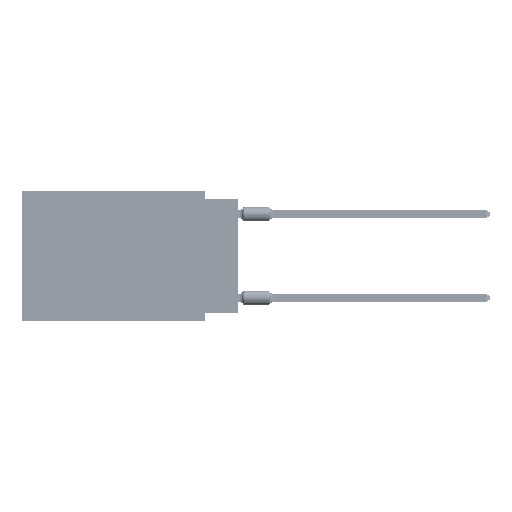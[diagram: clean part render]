
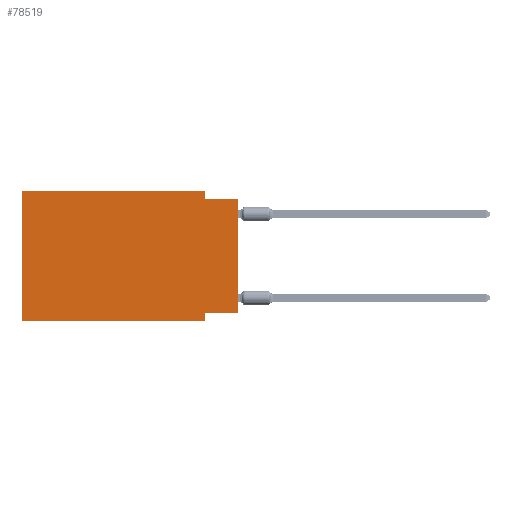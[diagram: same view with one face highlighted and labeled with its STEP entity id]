
A CAD part, left-side view. The second image highlights one B-rep face of the part: STEP entity #78519.
In plain terms, the highlighted planar face has unit normal (-1, 0, 0).
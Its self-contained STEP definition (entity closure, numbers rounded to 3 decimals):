
#569 = EDGE_CURVE ( 'NONE', #36816, #36761, #24789, .T. ) ;
#1434 = LINE ( 'NONE', #35737, #56379 ) ;
#3275 = DIRECTION ( 'NONE',  ( 0., 0., 1. ) ) ;
#5241 = DIRECTION ( 'NONE',  ( 0., 0., -1. ) ) ;
#5574 = ORIENTED_EDGE ( 'NONE', *, *, #16453, .F. ) ;
#5767 = CARTESIAN_POINT ( 'NONE',  ( 0., 0., -9.271 ) ) ;
#7867 = VERTEX_POINT ( 'NONE', #12869 ) ;
#8381 = CARTESIAN_POINT ( 'NONE',  ( 0., 0., -0.635 ) ) ;
#12153 = EDGE_LOOP ( 'NONE', ( #39560, #37066, #29864, #5574, #66683, #27872, #53788, #54369 ) ) ;
#12277 = FACE_OUTER_BOUND ( 'NONE', #12153, .T. ) ;
#12869 = CARTESIAN_POINT ( 'NONE',  ( 0., 16.383, 0. ) ) ;
#13129 = DIRECTION ( 'NONE',  ( 1., 0., 0. ) ) ;
#14637 = DIRECTION ( 'NONE',  ( 0., -1., 0. ) ) ;
#14796 = DIRECTION ( 'NONE',  ( 0., 0., -1. ) ) ;
#16453 = EDGE_CURVE ( 'NONE', #7867, #36816, #38893, .T. ) ;
#18211 = CARTESIAN_POINT ( 'NONE',  ( 0., 2.54, -0.635 ) ) ;
#20026 = EDGE_CURVE ( 'NONE', #57090, #71826, #1434, .T. ) ;
#21146 = CARTESIAN_POINT ( 'NONE',  ( 0., 2.54, -9.271 ) ) ;
#22377 = CARTESIAN_POINT ( 'NONE',  ( 0., 16.383, 0. ) ) ;
#23449 = LINE ( 'NONE', #74256, #75177 ) ;
#24789 = LINE ( 'NONE', #51705, #27773 ) ;
#25863 = CARTESIAN_POINT ( 'NONE',  ( 0., 0., -0.635 ) ) ;
#26068 = CARTESIAN_POINT ( 'NONE',  ( 0., 16.383, -9.906 ) ) ;
#27773 = VECTOR ( 'NONE', #5241, 1000. ) ;
#27872 = ORIENTED_EDGE ( 'NONE', *, *, #71903, .T. ) ;
#28178 = AXIS2_PLACEMENT_3D ( 'NONE', #47009, #13129, #39643 ) ;
#29864 = ORIENTED_EDGE ( 'NONE', *, *, #569, .F. ) ;
#30706 = VERTEX_POINT ( 'NONE', #61162 ) ;
#34869 = DIRECTION ( 'NONE',  ( 0., -1., 0. ) ) ;
#35737 = CARTESIAN_POINT ( 'NONE',  ( 0., 0., -9.271 ) ) ;
#36761 = VERTEX_POINT ( 'NONE', #18211 ) ;
#36816 = VERTEX_POINT ( 'NONE', #84238 ) ;
#37066 = ORIENTED_EDGE ( 'NONE', *, *, #48651, .F. ) ;
#38893 = LINE ( 'NONE', #46683, #54774 ) ;
#39560 = ORIENTED_EDGE ( 'NONE', *, *, #78697, .T. ) ;
#39643 = DIRECTION ( 'NONE',  ( 0., 0., -1. ) ) ;
#41404 = LINE ( 'NONE', #8381, #68779 ) ;
#46683 = CARTESIAN_POINT ( 'NONE',  ( 0., 16.383, 0. ) ) ;
#47009 = CARTESIAN_POINT ( 'NONE',  ( 0., 16.383, 0. ) ) ;
#48651 = EDGE_CURVE ( 'NONE', #36761, #57865, #41404, .T. ) ;
#49509 = VECTOR ( 'NONE', #14637, 1000. ) ;
#50766 = VERTEX_POINT ( 'NONE', #81956 ) ;
#51705 = CARTESIAN_POINT ( 'NONE',  ( 0., 2.54, 0. ) ) ;
#53397 = VECTOR ( 'NONE', #3275, 1000. ) ;
#53788 = ORIENTED_EDGE ( 'NONE', *, *, #67585, .F. ) ;
#54369 = ORIENTED_EDGE ( 'NONE', *, *, #20026, .F. ) ;
#54406 = DIRECTION ( 'NONE',  ( 0., 1., 0. ) ) ;
#54774 = VECTOR ( 'NONE', #65339, 1000. ) ;
#56379 = VECTOR ( 'NONE', #54406, 1000. ) ;
#57090 = VERTEX_POINT ( 'NONE', #5767 ) ;
#57865 = VERTEX_POINT ( 'NONE', #25863 ) ;
#60028 = VECTOR ( 'NONE', #74738, 1000. ) ;
#61162 = CARTESIAN_POINT ( 'NONE',  ( 0., 16.383, -9.906 ) ) ;
#65339 = DIRECTION ( 'NONE',  ( 0., -1., 0. ) ) ;
#66683 = ORIENTED_EDGE ( 'NONE', *, *, #69666, .F. ) ;
#67585 = EDGE_CURVE ( 'NONE', #71826, #50766, #23449, .T. ) ;
#68779 = VECTOR ( 'NONE', #34869, 1000. ) ;
#69105 = LINE ( 'NONE', #75166, #60028 ) ;
#69666 = EDGE_CURVE ( 'NONE', #30706, #7867, #81900, .T. ) ;
#71826 = VERTEX_POINT ( 'NONE', #21146 ) ;
#71903 = EDGE_CURVE ( 'NONE', #30706, #50766, #74107, .T. ) ;
#74107 = LINE ( 'NONE', #26068, #49509 ) ;
#74256 = CARTESIAN_POINT ( 'NONE',  ( 0., 2.54, -9.906 ) ) ;
#74738 = DIRECTION ( 'NONE',  ( 0., 0., 1. ) ) ;
#75166 = CARTESIAN_POINT ( 'NONE',  ( 0., 0., 0. ) ) ;
#75177 = VECTOR ( 'NONE', #14796, 1000. ) ;
#78519 = ADVANCED_FACE ( 'NONE', ( #12277 ), #79135, .F. ) ;
#78697 = EDGE_CURVE ( 'NONE', #57090, #57865, #69105, .T. ) ;
#79135 = PLANE ( 'NONE',  #28178 ) ;
#81900 = LINE ( 'NONE', #22377, #53397 ) ;
#81956 = CARTESIAN_POINT ( 'NONE',  ( 0., 2.54, -9.906 ) ) ;
#84238 = CARTESIAN_POINT ( 'NONE',  ( 0., 2.54, 0. ) ) ;
